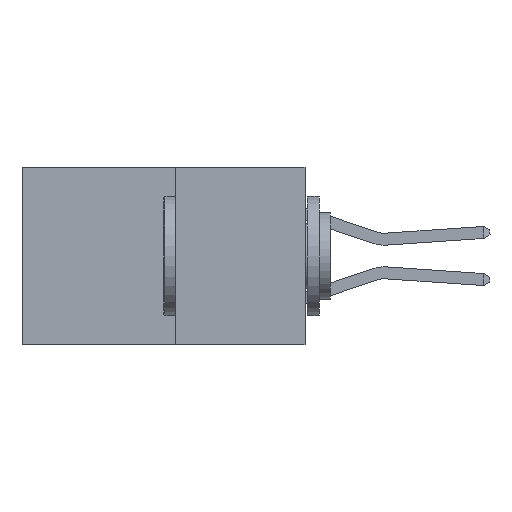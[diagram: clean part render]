
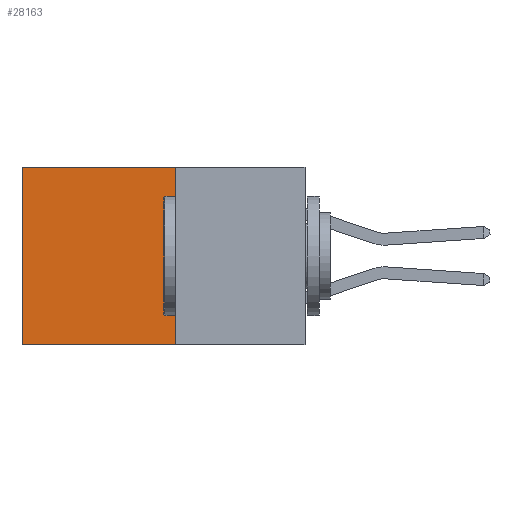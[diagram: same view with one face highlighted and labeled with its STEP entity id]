
A CAD part, left-side view. The second image highlights one B-rep face of the part: STEP entity #28163.
In plain terms, the highlighted planar face has unit normal (-1, 0, 0).
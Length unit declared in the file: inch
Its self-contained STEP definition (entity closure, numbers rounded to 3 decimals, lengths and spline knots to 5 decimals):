
#653 = VECTOR ( 'NONE', #13504, 39.37008 ) ;
#1005 = EDGE_CURVE ( 'NONE', #28300, #8916, #5726, .T. ) ;
#2011 = AXIS2_PLACEMENT_3D ( 'NONE', #11335, #27920, #13708 ) ;
#3663 = CARTESIAN_POINT ( 'NONE',  ( 0.277, 0.59, -0.37 ) ) ;
#3919 = ORIENTED_EDGE ( 'NONE', *, *, #20722, .T. ) ;
#4521 = EDGE_LOOP ( 'NONE', ( #3919, #6623, #20747, #11287 ) ) ;
#5726 = LINE ( 'NONE', #20241, #30241 ) ;
#5749 = VERTEX_POINT ( 'NONE', #5951 ) ;
#5951 = CARTESIAN_POINT ( 'NONE',  ( 0.277, 0.59, -0.37 ) ) ;
#6623 = ORIENTED_EDGE ( 'NONE', *, *, #22119, .F. ) ;
#6632 = DIRECTION ( 'NONE',  ( 0., 0., -1. ) ) ;
#8496 = VECTOR ( 'NONE', #25281, 39.37008 ) ;
#8916 = VERTEX_POINT ( 'NONE', #22676 ) ;
#9247 = LINE ( 'NONE', #27535, #8496 ) ;
#11123 = CARTESIAN_POINT ( 'NONE',  ( 0.277, 0.27, -0.37 ) ) ;
#11287 = ORIENTED_EDGE ( 'NONE', *, *, #14916, .T. ) ;
#11335 = CARTESIAN_POINT ( 'NONE',  ( 0.277, 0.27, -0.37 ) ) ;
#11858 = CARTESIAN_POINT ( 'NONE',  ( 0.277, 0.27, 0. ) ) ;
#13504 = DIRECTION ( 'NONE',  ( 0., 1., 0. ) ) ;
#13708 = DIRECTION ( 'NONE',  ( 0., 0., -1. ) ) ;
#14916 = EDGE_CURVE ( 'NONE', #28300, #17468, #9247, .T. ) ;
#15410 = FACE_OUTER_BOUND ( 'NONE', #4521, .T. ) ;
#17468 = VERTEX_POINT ( 'NONE', #27685 ) ;
#17985 = DIRECTION ( 'NONE',  ( 0., 0., -1. ) ) ;
#19359 = VECTOR ( 'NONE', #17985, 39.37008 ) ;
#19685 = LINE ( 'NONE', #11123, #653 ) ;
#20241 = CARTESIAN_POINT ( 'NONE',  ( 0.277, 0.27, -0.37 ) ) ;
#20722 = EDGE_CURVE ( 'NONE', #17468, #5749, #25680, .T. ) ;
#20747 = ORIENTED_EDGE ( 'NONE', *, *, #1005, .F. ) ;
#22119 = EDGE_CURVE ( 'NONE', #8916, #5749, #19685, .T. ) ;
#22676 = CARTESIAN_POINT ( 'NONE',  ( 0.277, 0.27, -0.37 ) ) ;
#25281 = DIRECTION ( 'NONE',  ( 0., 1., 0. ) ) ;
#25574 = PLANE ( 'NONE',  #2011 ) ;
#25680 = LINE ( 'NONE', #3663, #19359 ) ;
#27535 = CARTESIAN_POINT ( 'NONE',  ( 0.277, 0.27, 0. ) ) ;
#27685 = CARTESIAN_POINT ( 'NONE',  ( 0.277, 0.59, 0. ) ) ;
#27920 = DIRECTION ( 'NONE',  ( 1., 0., 0. ) ) ;
#28163 = ADVANCED_FACE ( 'NONE', ( #15410 ), #25574, .F. ) ;
#28300 = VERTEX_POINT ( 'NONE', #11858 ) ;
#30241 = VECTOR ( 'NONE', #6632, 39.37008 ) ;
